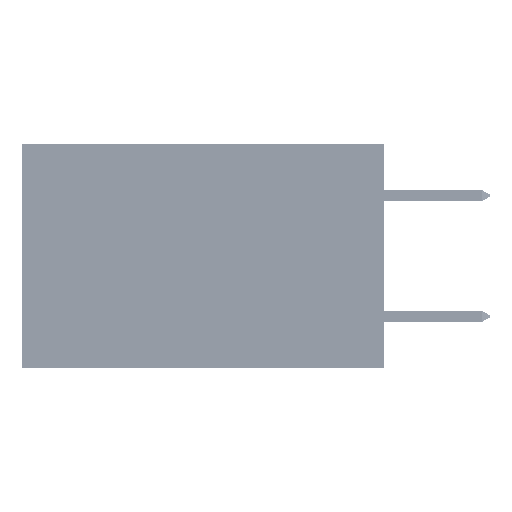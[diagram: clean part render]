
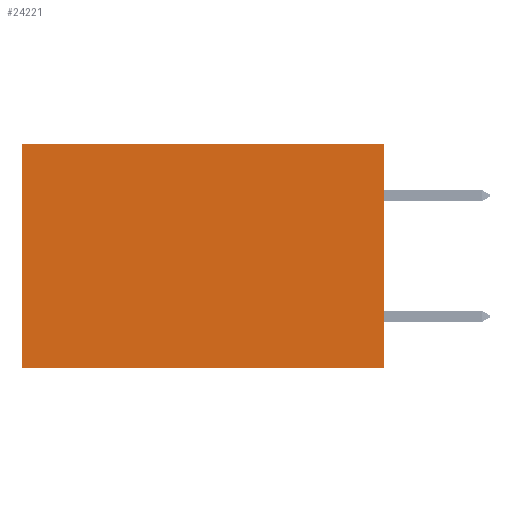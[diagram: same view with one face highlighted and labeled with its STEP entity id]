
A CAD part, left-side view. The second image highlights one B-rep face of the part: STEP entity #24221.
In plain terms, the highlighted planar face has unit normal (-1, 0, 0).
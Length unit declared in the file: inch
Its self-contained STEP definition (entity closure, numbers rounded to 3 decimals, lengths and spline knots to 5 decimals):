
#4618 = VERTEX_POINT ( 'NONE', #12301 ) ;
#5031 = CARTESIAN_POINT ( 'NONE',  ( 0.2875, 0.6, -0.37 ) ) ;
#5293 = DIRECTION ( 'NONE',  ( 0., 0., -1. ) ) ;
#6334 = DIRECTION ( 'NONE',  ( 0., 0., -1. ) ) ;
#6954 = VERTEX_POINT ( 'NONE', #9109 ) ;
#7771 = VECTOR ( 'NONE', #5293, 39.37008 ) ;
#8901 = EDGE_CURVE ( 'NONE', #6954, #44679, #12752, .T. ) ;
#9109 = CARTESIAN_POINT ( 'NONE',  ( 0.2875, 0., -0.37 ) ) ;
#10266 = VECTOR ( 'NONE', #14596, 39.37008 ) ;
#10427 = CARTESIAN_POINT ( 'NONE',  ( 0.2875, 0., -0.37 ) ) ;
#12088 = FACE_OUTER_BOUND ( 'NONE', #38530, .T. ) ;
#12301 = CARTESIAN_POINT ( 'NONE',  ( 0.2875, 0.6, 0. ) ) ;
#12752 = LINE ( 'NONE', #10427, #10266 ) ;
#13751 = CARTESIAN_POINT ( 'NONE',  ( 0.2875, 0., 0. ) ) ;
#14134 = DIRECTION ( 'NONE',  ( 1., 0., 0. ) ) ;
#14532 = VECTOR ( 'NONE', #29196, 39.37008 ) ;
#14596 = DIRECTION ( 'NONE',  ( 0., 1., 0. ) ) ;
#14797 = CARTESIAN_POINT ( 'NONE',  ( 0.2875, 0.6, 0. ) ) ;
#18411 = CARTESIAN_POINT ( 'NONE',  ( 0.2875, 0., 0. ) ) ;
#22720 = DIRECTION ( 'NONE',  ( 0., 0., -1. ) ) ;
#23042 = ORIENTED_EDGE ( 'NONE', *, *, #36221, .T. ) ;
#23068 = AXIS2_PLACEMENT_3D ( 'NONE', #18411, #14134, #6334 ) ;
#24077 = EDGE_CURVE ( 'NONE', #39663, #6954, #48460, .T. ) ;
#24221 = ADVANCED_FACE ( 'NONE', ( #12088 ), #30087, .F. ) ;
#24397 = EDGE_CURVE ( 'NONE', #4618, #44679, #39173, .T. ) ;
#28923 = ORIENTED_EDGE ( 'NONE', *, *, #24077, .F. ) ;
#29196 = DIRECTION ( 'NONE',  ( 0., 1., 0. ) ) ;
#30087 = PLANE ( 'NONE',  #23068 ) ;
#32303 = LINE ( 'NONE', #13751, #14532 ) ;
#32844 = CARTESIAN_POINT ( 'NONE',  ( 0.2875, 0., 0. ) ) ;
#34366 = ORIENTED_EDGE ( 'NONE', *, *, #24397, .T. ) ;
#36221 = EDGE_CURVE ( 'NONE', #39663, #4618, #32303, .T. ) ;
#37339 = VECTOR ( 'NONE', #22720, 39.37008 ) ;
#38530 = EDGE_LOOP ( 'NONE', ( #34366, #41633, #28923, #23042 ) ) ;
#39173 = LINE ( 'NONE', #14797, #37339 ) ;
#39663 = VERTEX_POINT ( 'NONE', #47728 ) ;
#41633 = ORIENTED_EDGE ( 'NONE', *, *, #8901, .F. ) ;
#44679 = VERTEX_POINT ( 'NONE', #5031 ) ;
#47728 = CARTESIAN_POINT ( 'NONE',  ( 0.2875, 0., 0. ) ) ;
#48460 = LINE ( 'NONE', #32844, #7771 ) ;
